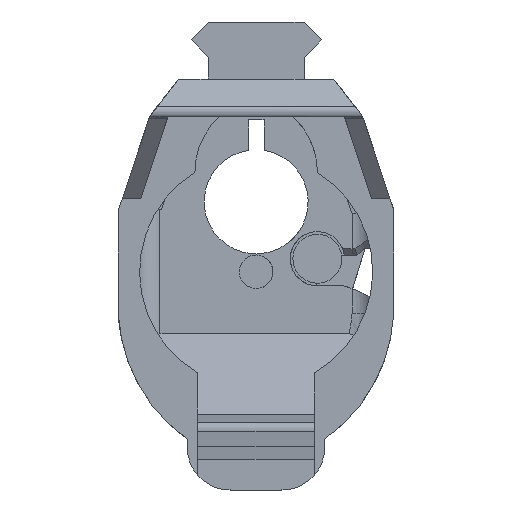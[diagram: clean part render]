
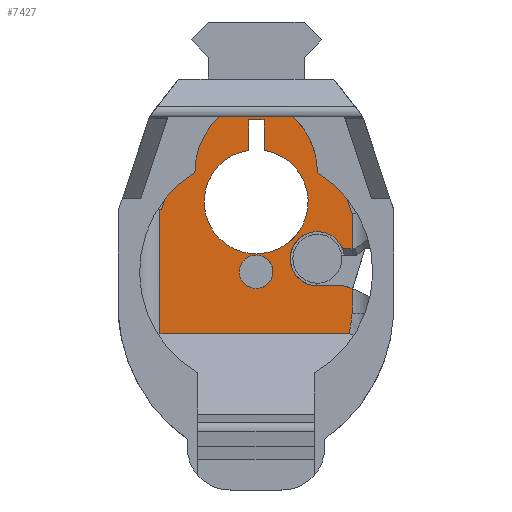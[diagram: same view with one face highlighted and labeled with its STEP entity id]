
A CAD part, front view. The second image highlights one B-rep face of the part: STEP entity #7427.
In plain terms, the highlighted planar face has unit normal (0, -1, 0).
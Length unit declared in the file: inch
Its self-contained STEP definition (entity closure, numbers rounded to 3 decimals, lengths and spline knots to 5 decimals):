
#20=FACE_BOUND('',#848,.T.);
#21=FACE_BOUND('',#849,.T.);
#107=CIRCLE('',#7807,0.17421);
#115=CIRCLE('',#7844,0.33465);
#119=CIRCLE('',#7854,0.10827);
#120=CIRCLE('',#7855,0.10827);
#130=CIRCLE('',#7953,0.78536);
#450=FACE_OUTER_BOUND('',#847,.T.);
#847=EDGE_LOOP('',(#5788,#5789,#5790,#5791,#5792,#5793,#5794,#5795,#5796,
#5797,#5798,#5799,#5800,#5801,#5802,#5803));
#848=EDGE_LOOP('',(#5804,#5805));
#849=EDGE_LOOP('',(#5806,#5807,#5808,#5809));
#1067=LINE('',#10200,#1994);
#1071=LINE('',#10209,#1998);
#1155=LINE('',#10491,#2082);
#1266=LINE('',#10816,#2193);
#1308=LINE('',#10921,#2235);
#1335=LINE('',#11025,#2262);
#1343=LINE('',#11058,#2270);
#1359=LINE('',#11162,#2286);
#1499=LINE('',#11579,#2426);
#1501=LINE('',#11582,#2428);
#1504=LINE('',#11623,#2431);
#1505=LINE('',#11626,#2432);
#1506=LINE('',#11629,#2433);
#1507=LINE('',#11631,#2434);
#1508=LINE('',#11633,#2435);
#1509=LINE('',#11635,#2436);
#1510=LINE('',#11636,#2437);
#1994=VECTOR('',#8216,0.3937);
#1998=VECTOR('',#8224,0.3937);
#2082=VECTOR('',#8420,0.3937);
#2193=VECTOR('',#8675,0.3937);
#2235=VECTOR('',#8757,0.3937);
#2262=VECTOR('',#8816,0.3937);
#2270=VECTOR('',#8838,0.3937);
#2286=VECTOR('',#8864,0.3937);
#2426=VECTOR('',#9222,0.3937);
#2428=VECTOR('',#9226,0.3937);
#2431=VECTOR('',#9243,0.3937);
#2432=VECTOR('',#9246,0.3937);
#2433=VECTOR('',#9251,0.3937);
#2434=VECTOR('',#9252,0.3937);
#2435=VECTOR('',#9255,0.3937);
#2436=VECTOR('',#9256,0.3937);
#2437=VECTOR('',#9257,0.3937);
#2921=VERTEX_POINT('',#10197);
#2922=VERTEX_POINT('',#10199);
#2925=VERTEX_POINT('',#10207);
#3011=VERTEX_POINT('',#10489);
#3110=VERTEX_POINT('',#10815);
#3152=VERTEX_POINT('',#10918);
#3153=VERTEX_POINT('',#10920);
#3156=VERTEX_POINT('',#10928);
#3172=VERTEX_POINT('',#11022);
#3173=VERTEX_POINT('',#11024);
#3184=VERTEX_POINT('',#11055);
#3185=VERTEX_POINT('',#11057);
#3200=VERTEX_POINT('',#11160);
#3218=VERTEX_POINT('',#11208);
#3219=VERTEX_POINT('',#11210);
#3236=VERTEX_POINT('',#11288);
#3237=VERTEX_POINT('',#11289);
#3302=VERTEX_POINT('',#11578);
#3307=VERTEX_POINT('',#11621);
#3308=VERTEX_POINT('',#11625);
#3309=VERTEX_POINT('',#11630);
#3310=VERTEX_POINT('',#11634);
#3626=EDGE_CURVE('',#2921,#2922,#1067,.T.);
#3631=EDGE_CURVE('',#2921,#2925,#1071,.T.);
#3748=EDGE_CURVE('',#2925,#3011,#1155,.T.);
#3892=EDGE_CURVE('',#3110,#2922,#1266,.T.);
#3943=EDGE_CURVE('',#3153,#3152,#1308,.T.);
#3948=EDGE_CURVE('',#3152,#3156,#107,.T.);
#3978=EDGE_CURVE('',#3172,#3173,#1335,.T.);
#3992=EDGE_CURVE('',#3184,#3185,#1343,.T.);
#4015=EDGE_CURVE('',#3200,#3156,#1359,.T.);
#4038=EDGE_CURVE('',#3219,#3218,#115,.T.);
#4059=EDGE_CURVE('',#3236,#3237,#119,.T.);
#4060=EDGE_CURVE('',#3237,#3236,#120,.T.);
#4200=EDGE_CURVE('',#3302,#3219,#1499,.T.);
#4202=EDGE_CURVE('',#3173,#3011,#1501,.T.);
#4211=EDGE_CURVE('',#3307,#3172,#1504,.T.);
#4212=EDGE_CURVE('',#3110,#3308,#1505,.T.);
#4214=EDGE_CURVE('',#3308,#3200,#1506,.T.);
#4215=EDGE_CURVE('',#3307,#3309,#1507,.T.);
#4216=EDGE_CURVE('',#3185,#3309,#130,.T.);
#4217=EDGE_CURVE('',#3153,#3184,#1508,.T.);
#4218=EDGE_CURVE('',#3218,#3310,#1509,.T.);
#4219=EDGE_CURVE('',#3310,#3302,#1510,.T.);
#5788=ORIENTED_EDGE('',*,*,#4015,.F.);
#5789=ORIENTED_EDGE('',*,*,#4214,.F.);
#5790=ORIENTED_EDGE('',*,*,#4212,.F.);
#5791=ORIENTED_EDGE('',*,*,#3892,.T.);
#5792=ORIENTED_EDGE('',*,*,#3626,.F.);
#5793=ORIENTED_EDGE('',*,*,#3631,.T.);
#5794=ORIENTED_EDGE('',*,*,#3748,.T.);
#5795=ORIENTED_EDGE('',*,*,#4202,.F.);
#5796=ORIENTED_EDGE('',*,*,#3978,.F.);
#5797=ORIENTED_EDGE('',*,*,#4211,.F.);
#5798=ORIENTED_EDGE('',*,*,#4215,.T.);
#5799=ORIENTED_EDGE('',*,*,#4216,.F.);
#5800=ORIENTED_EDGE('',*,*,#3992,.F.);
#5801=ORIENTED_EDGE('',*,*,#4217,.F.);
#5802=ORIENTED_EDGE('',*,*,#3943,.T.);
#5803=ORIENTED_EDGE('',*,*,#3948,.T.);
#5804=ORIENTED_EDGE('',*,*,#4059,.T.);
#5805=ORIENTED_EDGE('',*,*,#4060,.T.);
#5806=ORIENTED_EDGE('',*,*,#4200,.T.);
#5807=ORIENTED_EDGE('',*,*,#4038,.T.);
#5808=ORIENTED_EDGE('',*,*,#4218,.T.);
#5809=ORIENTED_EDGE('',*,*,#4219,.T.);
#7049=PLANE('',#7952);
#7427=ADVANCED_FACE('',(#450,#20,#21),#7049,.T.);
#7807=AXIS2_PLACEMENT_3D('',#10930,#8765,#8766);
#7844=AXIS2_PLACEMENT_3D('',#11211,#8902,#8903);
#7854=AXIS2_PLACEMENT_3D('',#11290,#8937,#8938);
#7855=AXIS2_PLACEMENT_3D('',#11291,#8939,#8940);
#7952=AXIS2_PLACEMENT_3D('',#11628,#9249,#9250);
#7953=AXIS2_PLACEMENT_3D('',#11632,#9253,#9254);
#8216=DIRECTION('',(1.,0.,-0.002));
#8224=DIRECTION('',(0.,0.,-1.));
#8420=DIRECTION('',(-1.,0.,0.));
#8675=DIRECTION('',(0.002,0.,1.));
#8757=DIRECTION('',(-1.,0.,0.));
#8765=DIRECTION('center_axis',(0.,1.,0.));
#8766=DIRECTION('ref_axis',(1.,0.,0.));
#8816=DIRECTION('',(1.,0.,0.));
#8838=DIRECTION('',(0.,0.,-1.));
#8864=DIRECTION('',(-1.,0.,0.));
#8902=DIRECTION('center_axis',(0.,1.,0.));
#8903=DIRECTION('ref_axis',(-1.,0.,0.));
#8937=DIRECTION('center_axis',(0.,1.,0.));
#8938=DIRECTION('ref_axis',(1.,0.,0.));
#8939=DIRECTION('center_axis',(0.,1.,0.));
#8940=DIRECTION('ref_axis',(1.,0.,0.));
#9222=DIRECTION('',(0.,0.,-1.));
#9226=DIRECTION('',(0.316,0.,0.949));
#9243=DIRECTION('',(0.,0.,1.));
#9246=DIRECTION('',(0.316,0.,-0.949));
#9249=DIRECTION('center_axis',(0.,-1.,0.));
#9250=DIRECTION('ref_axis',(0.,0.,-1.));
#9251=DIRECTION('',(0.,0.,-1.));
#9252=DIRECTION('',(1.,0.,0.));
#9253=DIRECTION('center_axis',(0.,1.,0.));
#9254=DIRECTION('ref_axis',(0.992,0.,-0.128));
#9255=DIRECTION('',(0.954,0.,-0.301));
#9256=DIRECTION('',(0.,0.,1.));
#9257=DIRECTION('',(1.,0.,0.));
#10197=CARTESIAN_POINT('',(0.5,2.56,1.0001));
#10199=CARTESIAN_POINT('',(0.56627,2.56,0.99997));
#10200=CARTESIAN_POINT('',(0.5,2.56,1.0001));
#10207=CARTESIAN_POINT('',(0.5,2.56,0.99982));
#10209=CARTESIAN_POINT('',(0.5,2.56,0.64988));
#10489=CARTESIAN_POINT('',(-0.40817,2.56,0.99982));
#10491=CARTESIAN_POINT('',(-0.5,2.56,0.99982));
#10815=CARTESIAN_POINT('',(0.56534,2.56,0.52831));
#10816=CARTESIAN_POINT('',(0.56627,2.56,0.99987));
#10918=CARTESIAN_POINT('',(0.41433,2.56,-0.08921));
#10920=CARTESIAN_POINT('',(0.55783,2.56,-0.08921));
#10921=CARTESIAN_POINT('',(0.10264,2.56,-0.08921));
#10928=CARTESIAN_POINT('',(0.55575,2.56,0.14773));
#10930=CARTESIAN_POINT('Origin',(0.3937,2.56,0.08378));
#11022=CARTESIAN_POINT('',(-0.61864,2.56,0.39831));
#11024=CARTESIAN_POINT('',(-0.60868,2.56,0.39831));
#11025=CARTESIAN_POINT('',(-0.79245,2.56,0.39831));
#11055=CARTESIAN_POINT('',(0.61679,2.56,-0.1078));
#11057=CARTESIAN_POINT('',(0.61679,2.56,-0.26638));
#11058=CARTESIAN_POINT('',(0.61679,2.56,0.01448));
#11160=CARTESIAN_POINT('',(0.61679,2.56,0.14773));
#11162=CARTESIAN_POINT('',(0.03313,2.56,0.14773));
#11208=CARTESIAN_POINT('',(-0.0477,2.56,0.78123));
#11210=CARTESIAN_POINT('',(0.05072,2.56,0.78078));
#11211=CARTESIAN_POINT('Origin',(0.,2.56,0.45));
#11288=CARTESIAN_POINT('',(-0.05174,2.56,0.0951));
#11289=CARTESIAN_POINT('',(-0.10827,2.56,0.));
#11290=CARTESIAN_POINT('Origin',(0.,2.56,0.));
#11291=CARTESIAN_POINT('Origin',(0.,2.56,0.));
#11578=CARTESIAN_POINT('',(0.05072,2.56,0.97719));
#11579=CARTESIAN_POINT('',(0.05072,2.56,0.54014));
#11582=CARTESIAN_POINT('',(-0.6259,2.56,0.34662));
#11621=CARTESIAN_POINT('',(-0.61864,2.56,-0.4));
#11623=CARTESIAN_POINT('',(-0.61864,2.56,0.34912));
#11625=CARTESIAN_POINT('',(0.61679,2.56,0.37396));
#11626=CARTESIAN_POINT('',(0.47564,2.56,0.79741));
#11628=CARTESIAN_POINT('Origin',(-0.5,2.56,0.29994));
#11629=CARTESIAN_POINT('',(0.61679,2.56,0.01448));
#11630=CARTESIAN_POINT('',(0.59654,2.56,-0.4));
#11631=CARTESIAN_POINT('',(0.37309,2.56,-0.4));
#11632=CARTESIAN_POINT('Origin',(-0.16695,2.56,-0.21593));
#11633=CARTESIAN_POINT('',(0.05278,2.56,0.07004));
#11634=CARTESIAN_POINT('',(-0.0477,2.56,0.97719));
#11635=CARTESIAN_POINT('',(-0.0477,2.56,0.54014));
#11636=CARTESIAN_POINT('',(-0.22464,2.56,0.97719));
